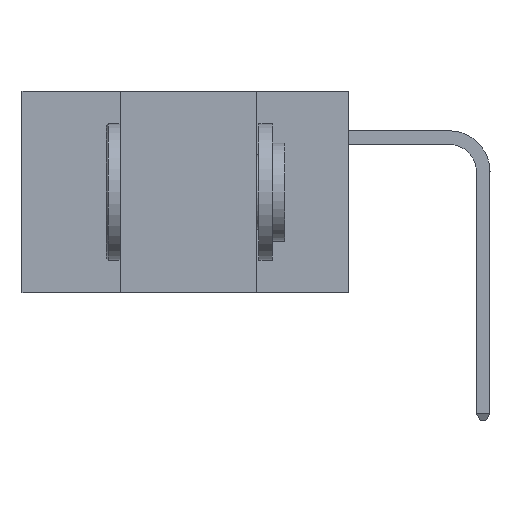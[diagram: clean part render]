
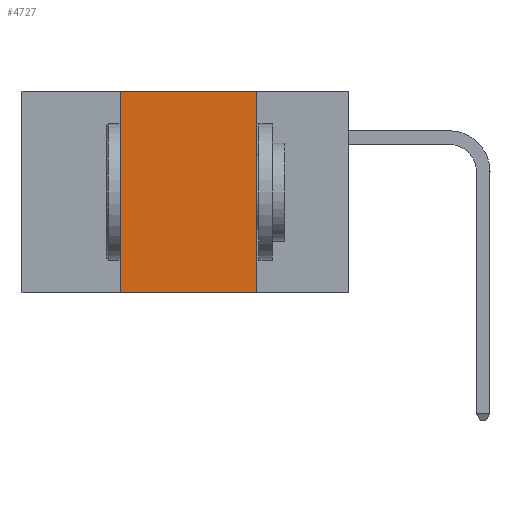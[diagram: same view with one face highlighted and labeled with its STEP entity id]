
A CAD part, left-side view. The second image highlights one B-rep face of the part: STEP entity #4727.
In plain terms, the highlighted planar face has unit normal (-1, 0, 0).
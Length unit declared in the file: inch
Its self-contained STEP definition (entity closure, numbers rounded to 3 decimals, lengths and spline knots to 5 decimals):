
#205 = DIRECTION ( 'NONE',  ( 0., 0., -1. ) ) ;
#234 = DIRECTION ( 'NONE',  ( 1., 0., 0. ) ) ;
#257 = CARTESIAN_POINT ( 'NONE',  ( 0., 0.6, 0. ) ) ;
#314 = VECTOR ( 'NONE', #6894, 39.37008 ) ;
#835 = ORIENTED_EDGE ( 'NONE', *, *, #7747, .F. ) ;
#1302 = VERTEX_POINT ( 'NONE', #12820 ) ;
#1485 = EDGE_LOOP ( 'NONE', ( #835, #8305, #15209, #5491 ) ) ;
#1633 = VECTOR ( 'NONE', #9575, 39.37008 ) ;
#1941 = LINE ( 'NONE', #4720, #15028 ) ;
#2387 = CARTESIAN_POINT ( 'NONE',  ( 0., 0.42, 0. ) ) ;
#3040 = AXIS2_PLACEMENT_3D ( 'NONE', #257, #234, #205 ) ;
#3106 = CARTESIAN_POINT ( 'NONE',  ( 0., 0.17, -0.37 ) ) ;
#3326 = PLANE ( 'NONE',  #3040 ) ;
#4251 = CARTESIAN_POINT ( 'NONE',  ( 0., 0.6, -0.37 ) ) ;
#4720 = CARTESIAN_POINT ( 'NONE',  ( 0., 0.17, 0. ) ) ;
#4727 = ADVANCED_FACE ( 'NONE', ( #16124 ), #3326, .F. ) ;
#5128 = EDGE_CURVE ( 'NONE', #1302, #8556, #5187, .T. ) ;
#5187 = LINE ( 'NONE', #13910, #1633 ) ;
#5491 = ORIENTED_EDGE ( 'NONE', *, *, #12453, .T. ) ;
#5589 = CARTESIAN_POINT ( 'NONE',  ( 0., 0.6, 0. ) ) ;
#6360 = LINE ( 'NONE', #5589, #12887 ) ;
#6821 = EDGE_CURVE ( 'NONE', #8556, #12087, #6360, .T. ) ;
#6894 = DIRECTION ( 'NONE',  ( 0., -1., 0. ) ) ;
#6903 = DIRECTION ( 'NONE',  ( 0., -1., 0. ) ) ;
#7747 = EDGE_CURVE ( 'NONE', #12087, #15265, #1941, .T. ) ;
#8305 = ORIENTED_EDGE ( 'NONE', *, *, #6821, .F. ) ;
#8547 = DIRECTION ( 'NONE',  ( 0., 0., -1. ) ) ;
#8556 = VERTEX_POINT ( 'NONE', #2387 ) ;
#8810 = CARTESIAN_POINT ( 'NONE',  ( 0., 0.17, 0. ) ) ;
#9575 = DIRECTION ( 'NONE',  ( 0., 0., 1. ) ) ;
#12087 = VERTEX_POINT ( 'NONE', #8810 ) ;
#12453 = EDGE_CURVE ( 'NONE', #1302, #15265, #14783, .T. ) ;
#12820 = CARTESIAN_POINT ( 'NONE',  ( 0., 0.42, -0.37 ) ) ;
#12887 = VECTOR ( 'NONE', #6903, 39.37008 ) ;
#13910 = CARTESIAN_POINT ( 'NONE',  ( 0., 0.42, 0. ) ) ;
#14783 = LINE ( 'NONE', #4251, #314 ) ;
#15028 = VECTOR ( 'NONE', #8547, 39.37008 ) ;
#15209 = ORIENTED_EDGE ( 'NONE', *, *, #5128, .F. ) ;
#15265 = VERTEX_POINT ( 'NONE', #3106 ) ;
#16124 = FACE_OUTER_BOUND ( 'NONE', #1485, .T. ) ;
